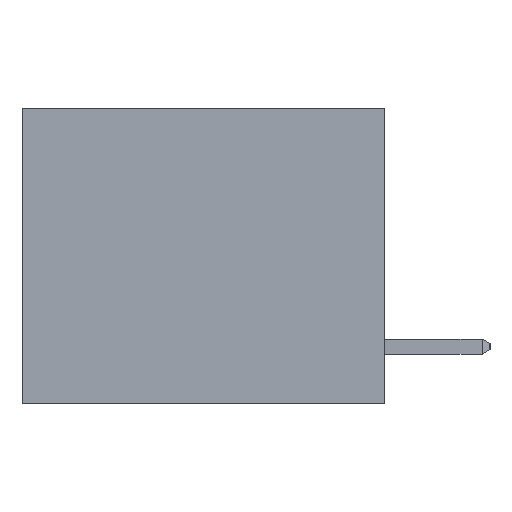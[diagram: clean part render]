
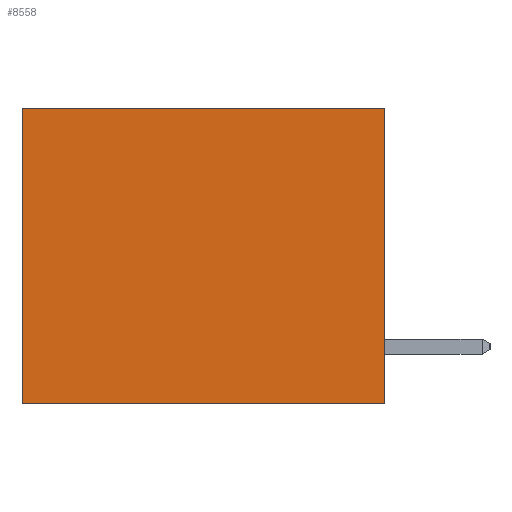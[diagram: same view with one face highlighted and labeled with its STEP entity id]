
A CAD part, left-side view. The second image highlights one B-rep face of the part: STEP entity #8558.
In plain terms, the highlighted planar face has unit normal (-1, 0, 0).
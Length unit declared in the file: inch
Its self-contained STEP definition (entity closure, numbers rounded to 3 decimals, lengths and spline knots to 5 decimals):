
#601 = ORIENTED_EDGE ( 'NONE', *, *, #12412, .T. ) ;
#1454 = DIRECTION ( 'NONE',  ( 0., 0., -1. ) ) ;
#2154 = EDGE_LOOP ( 'NONE', ( #601, #6824, #3613, #14113 ) ) ;
#2401 = VECTOR ( 'NONE', #17659, 39.37008 ) ;
#2502 = EDGE_CURVE ( 'NONE', #15188, #7650, #13814, .T. ) ;
#2961 = DIRECTION ( 'NONE',  ( 0., 0., -1. ) ) ;
#3600 = FACE_OUTER_BOUND ( 'NONE', #2154, .T. ) ;
#3613 = ORIENTED_EDGE ( 'NONE', *, *, #2502, .F. ) ;
#3990 = CARTESIAN_POINT ( 'NONE',  ( 0.3165, 0., -0.49 ) ) ;
#6722 = EDGE_CURVE ( 'NONE', #7650, #17960, #19923, .T. ) ;
#6824 = ORIENTED_EDGE ( 'NONE', *, *, #6722, .F. ) ;
#7053 = DIRECTION ( 'NONE',  ( 0., 0., -1. ) ) ;
#7242 = CARTESIAN_POINT ( 'NONE',  ( 0.3165, 0., 0. ) ) ;
#7650 = VERTEX_POINT ( 'NONE', #12685 ) ;
#7673 = VERTEX_POINT ( 'NONE', #8133 ) ;
#8133 = CARTESIAN_POINT ( 'NONE',  ( 0.3165, 0.6, 0. ) ) ;
#8558 = ADVANCED_FACE ( 'NONE', ( #3600 ), #15125, .F. ) ;
#9013 = AXIS2_PLACEMENT_3D ( 'NONE', #18446, #13580, #2961 ) ;
#10854 = CARTESIAN_POINT ( 'NONE',  ( 0.3165, 0.6, -0.49 ) ) ;
#12283 = CARTESIAN_POINT ( 'NONE',  ( 0.3165, 0., 0. ) ) ;
#12412 = EDGE_CURVE ( 'NONE', #7673, #17960, #13061, .T. ) ;
#12685 = CARTESIAN_POINT ( 'NONE',  ( 0.3165, 0., -0.49 ) ) ;
#13061 = LINE ( 'NONE', #10854, #19349 ) ;
#13580 = DIRECTION ( 'NONE',  ( 1., 0., 0. ) ) ;
#13756 = VECTOR ( 'NONE', #18110, 39.37008 ) ;
#13814 = LINE ( 'NONE', #3990, #15969 ) ;
#14113 = ORIENTED_EDGE ( 'NONE', *, *, #14198, .T. ) ;
#14198 = EDGE_CURVE ( 'NONE', #15188, #7673, #20080, .T. ) ;
#15125 = PLANE ( 'NONE',  #9013 ) ;
#15188 = VERTEX_POINT ( 'NONE', #12283 ) ;
#15969 = VECTOR ( 'NONE', #7053, 39.37008 ) ;
#16071 = CARTESIAN_POINT ( 'NONE',  ( 0.3165, 0., -0.49 ) ) ;
#16428 = CARTESIAN_POINT ( 'NONE',  ( 0.3165, 0.6, -0.49 ) ) ;
#17659 = DIRECTION ( 'NONE',  ( 0., 1., 0. ) ) ;
#17960 = VERTEX_POINT ( 'NONE', #16428 ) ;
#18110 = DIRECTION ( 'NONE',  ( 0., 1., 0. ) ) ;
#18446 = CARTESIAN_POINT ( 'NONE',  ( 0.3165, 0., -0.49 ) ) ;
#19349 = VECTOR ( 'NONE', #1454, 39.37008 ) ;
#19923 = LINE ( 'NONE', #16071, #2401 ) ;
#20080 = LINE ( 'NONE', #7242, #13756 ) ;
